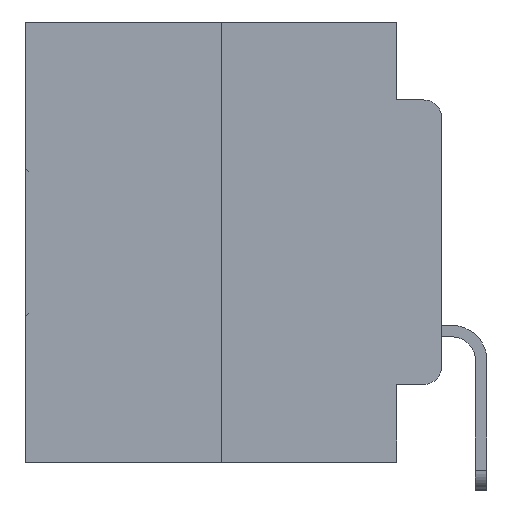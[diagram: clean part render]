
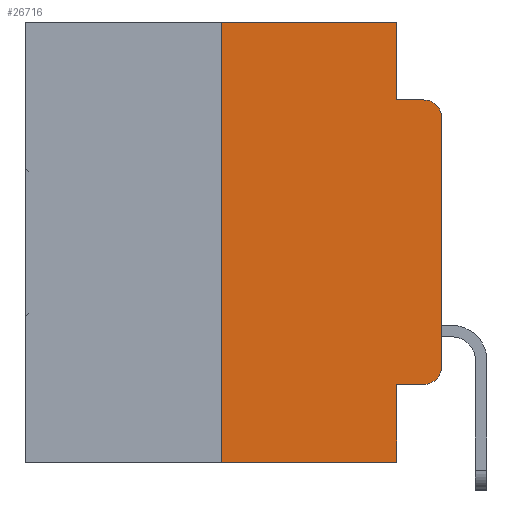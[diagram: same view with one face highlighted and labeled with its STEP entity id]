
A CAD part, left-side view. The second image highlights one B-rep face of the part: STEP entity #26716.
In plain terms, the highlighted planar face has unit normal (-1, 0, 0).
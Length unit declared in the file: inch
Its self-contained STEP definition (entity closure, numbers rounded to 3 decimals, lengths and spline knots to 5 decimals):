
#91 = CARTESIAN_POINT ( 'NONE',  ( 0., 0.02, -0.0885 ) ) ;
#105 = AXIS2_PLACEMENT_3D ( 'NONE', #12753, #28334, #15125 ) ;
#269 = VERTEX_POINT ( 'NONE', #8872 ) ;
#1228 = LINE ( 'NONE', #12145, #13616 ) ;
#2129 = EDGE_CURVE ( 'NONE', #15390, #23584, #7443, .T. ) ;
#2607 = LINE ( 'NONE', #2949, #14834 ) ;
#2949 = CARTESIAN_POINT ( 'NONE',  ( 0., 0.473, 0. ) ) ;
#3785 = EDGE_LOOP ( 'NONE', ( #13287, #14220, #15414, #15435, #16044, #16219, #16461, #16862, #16898, #17033 ) ) ;
#3959 = EDGE_CURVE ( 'NONE', #14175, #6445, #1228, .T. ) ;
#4905 = DIRECTION ( 'NONE',  ( 0., 0., -1. ) ) ;
#5429 = CARTESIAN_POINT ( 'NONE',  ( 0., 0.051, 0. ) ) ;
#6163 = VECTOR ( 'NONE', #30000, 39.37008 ) ;
#6445 = VERTEX_POINT ( 'NONE', #8133 ) ;
#6650 = FACE_OUTER_BOUND ( 'NONE', #3785, .T. ) ;
#6975 = DIRECTION ( 'NONE',  ( 0., -1., 0. ) ) ;
#6977 = VERTEX_POINT ( 'NONE', #28386 ) ;
#7443 = CIRCLE ( 'NONE', #25142, 0.02 ) ;
#7473 = AXIS2_PLACEMENT_3D ( 'NONE', #27799, #25714, #12227 ) ;
#8054 = CARTESIAN_POINT ( 'NONE',  ( 0., 0.25, 0. ) ) ;
#8133 = CARTESIAN_POINT ( 'NONE',  ( 0., 0.051, -0.0885 ) ) ;
#8813 = EDGE_CURVE ( 'NONE', #14608, #22114, #12856, .T. ) ;
#8872 = CARTESIAN_POINT ( 'NONE',  ( 0., 0.051, -0.4115 ) ) ;
#9260 = CARTESIAN_POINT ( 'NONE',  ( 0., 0., -0.1085 ) ) ;
#9720 = CARTESIAN_POINT ( 'NONE',  ( 0., 0.02, -0.4115 ) ) ;
#10040 = VECTOR ( 'NONE', #29750, 39.37008 ) ;
#10413 = DIRECTION ( 'NONE',  ( -1., 0., 0. ) ) ;
#10922 = CARTESIAN_POINT ( 'NONE',  ( 0., 0.02, -0.1085 ) ) ;
#11055 = VERTEX_POINT ( 'NONE', #12356 ) ;
#12145 = CARTESIAN_POINT ( 'NONE',  ( 0., 0.051, 0. ) ) ;
#12227 = DIRECTION ( 'NONE',  ( 0., 0., -1. ) ) ;
#12333 = LINE ( 'NONE', #8054, #29338 ) ;
#12346 = CARTESIAN_POINT ( 'NONE',  ( 0., 0.051, -0.5 ) ) ;
#12356 = CARTESIAN_POINT ( 'NONE',  ( 0., 0.25, 0. ) ) ;
#12753 = CARTESIAN_POINT ( 'NONE',  ( 0., 0.02, -0.3915 ) ) ;
#12856 = LINE ( 'NONE', #23264, #23510 ) ;
#12945 = LINE ( 'NONE', #28791, #13680 ) ;
#12996 = EDGE_CURVE ( 'NONE', #11055, #14175, #2607, .T. ) ;
#13287 = ORIENTED_EDGE ( 'NONE', *, *, #21844, .T. ) ;
#13292 = DIRECTION ( 'NONE',  ( 0., -1., 0. ) ) ;
#13316 = LINE ( 'NONE', #27926, #6163 ) ;
#13616 = VECTOR ( 'NONE', #4905, 39.37008 ) ;
#13668 = EDGE_CURVE ( 'NONE', #6445, #23584, #12945, .T. ) ;
#13680 = VECTOR ( 'NONE', #13292, 39.37008 ) ;
#14013 = CARTESIAN_POINT ( 'NONE',  ( 0., 0., 0. ) ) ;
#14175 = VERTEX_POINT ( 'NONE', #5429 ) ;
#14220 = ORIENTED_EDGE ( 'NONE', *, *, #2129, .T. ) ;
#14608 = VERTEX_POINT ( 'NONE', #29827 ) ;
#14834 = VECTOR ( 'NONE', #28304, 39.37008 ) ;
#15125 = DIRECTION ( 'NONE',  ( 0., 0., -1. ) ) ;
#15390 = VERTEX_POINT ( 'NONE', #9260 ) ;
#15414 = ORIENTED_EDGE ( 'NONE', *, *, #13668, .F. ) ;
#15435 = ORIENTED_EDGE ( 'NONE', *, *, #3959, .F. ) ;
#16044 = ORIENTED_EDGE ( 'NONE', *, *, #12996, .F. ) ;
#16219 = ORIENTED_EDGE ( 'NONE', *, *, #26278, .F. ) ;
#16461 = ORIENTED_EDGE ( 'NONE', *, *, #8813, .T. ) ;
#16738 = CARTESIAN_POINT ( 'NONE',  ( 0., 0.051, 0. ) ) ;
#16862 = ORIENTED_EDGE ( 'NONE', *, *, #18321, .F. ) ;
#16898 = ORIENTED_EDGE ( 'NONE', *, *, #29997, .T. ) ;
#17033 = ORIENTED_EDGE ( 'NONE', *, *, #24301, .T. ) ;
#18321 = EDGE_CURVE ( 'NONE', #269, #22114, #21603, .T. ) ;
#21603 = LINE ( 'NONE', #16738, #10040 ) ;
#21844 = EDGE_CURVE ( 'NONE', #6977, #15390, #29465, .T. ) ;
#22114 = VERTEX_POINT ( 'NONE', #12346 ) ;
#22995 = DIRECTION ( 'NONE',  ( 0., 0., 1. ) ) ;
#23141 = VECTOR ( 'NONE', #22995, 39.37008 ) ;
#23264 = CARTESIAN_POINT ( 'NONE',  ( 0., 0.473, -0.5 ) ) ;
#23510 = VECTOR ( 'NONE', #6975, 39.37008 ) ;
#23584 = VERTEX_POINT ( 'NONE', #91 ) ;
#24038 = DIRECTION ( 'NONE',  ( 0., 0., 1. ) ) ;
#24179 = VERTEX_POINT ( 'NONE', #9720 ) ;
#24301 = EDGE_CURVE ( 'NONE', #24179, #6977, #28679, .T. ) ;
#24598 = DIRECTION ( 'NONE',  ( 0., 0., -1. ) ) ;
#25142 = AXIS2_PLACEMENT_3D ( 'NONE', #10922, #10413, #24598 ) ;
#25624 = PLANE ( 'NONE',  #7473 ) ;
#25714 = DIRECTION ( 'NONE',  ( 1., 0., 0. ) ) ;
#26278 = EDGE_CURVE ( 'NONE', #14608, #11055, #12333, .T. ) ;
#26716 = ADVANCED_FACE ( 'NONE', ( #6650 ), #25624, .F. ) ;
#27799 = CARTESIAN_POINT ( 'NONE',  ( 0., 0.473, 0. ) ) ;
#27926 = CARTESIAN_POINT ( 'NONE',  ( 0., 0.051, -0.4115 ) ) ;
#28304 = DIRECTION ( 'NONE',  ( 0., -1., 0. ) ) ;
#28334 = DIRECTION ( 'NONE',  ( -1., 0., 0. ) ) ;
#28386 = CARTESIAN_POINT ( 'NONE',  ( 0., 0., -0.3915 ) ) ;
#28679 = CIRCLE ( 'NONE', #105, 0.02 ) ;
#28791 = CARTESIAN_POINT ( 'NONE',  ( 0., 0.051, -0.0885 ) ) ;
#29338 = VECTOR ( 'NONE', #24038, 39.37008 ) ;
#29465 = LINE ( 'NONE', #14013, #23141 ) ;
#29750 = DIRECTION ( 'NONE',  ( 0., 0., -1. ) ) ;
#29827 = CARTESIAN_POINT ( 'NONE',  ( 0., 0.25, -0.5 ) ) ;
#29997 = EDGE_CURVE ( 'NONE', #269, #24179, #13316, .T. ) ;
#30000 = DIRECTION ( 'NONE',  ( 0., -1., 0. ) ) ;
